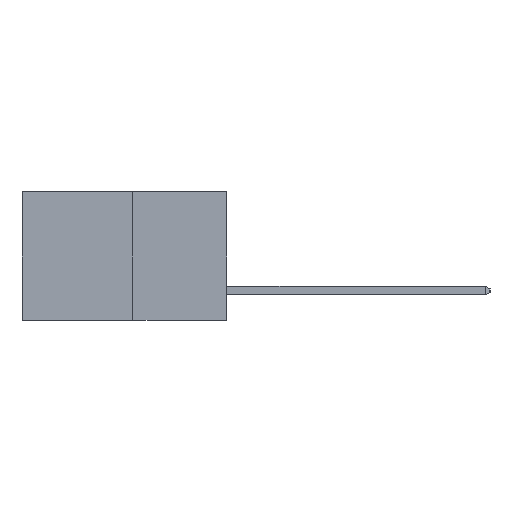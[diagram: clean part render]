
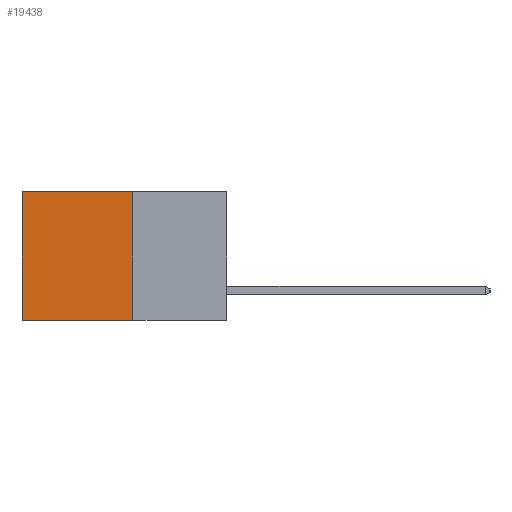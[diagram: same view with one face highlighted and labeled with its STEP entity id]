
A CAD part, left-side view. The second image highlights one B-rep face of the part: STEP entity #19438.
In plain terms, the highlighted planar face has unit normal (-1, 0, 0).
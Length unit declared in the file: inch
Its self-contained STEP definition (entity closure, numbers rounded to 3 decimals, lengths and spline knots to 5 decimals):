
#30 = DIRECTION ( 'NONE',  ( 0., 0., -1. ) ) ;
#348 = DIRECTION ( 'NONE',  ( 0., 1., 0. ) ) ;
#1043 = EDGE_LOOP ( 'NONE', ( #12575, #23502, #5970, #2455 ) ) ;
#2455 = ORIENTED_EDGE ( 'NONE', *, *, #4998, .T. ) ;
#3091 = LINE ( 'NONE', #18232, #7627 ) ;
#3432 = AXIS2_PLACEMENT_3D ( 'NONE', #16353, #6871, #20139 ) ;
#4824 = DIRECTION ( 'NONE',  ( 0., 0., -1. ) ) ;
#4951 = LINE ( 'NONE', #11866, #10711 ) ;
#4998 = EDGE_CURVE ( 'NONE', #17499, #17588, #3091, .T. ) ;
#5282 = EDGE_CURVE ( 'NONE', #17588, #18586, #11205, .T. ) ;
#5970 = ORIENTED_EDGE ( 'NONE', *, *, #10789, .F. ) ;
#6871 = DIRECTION ( 'NONE',  ( 1., 0., 0. ) ) ;
#7493 = VERTEX_POINT ( 'NONE', #19551 ) ;
#7627 = VECTOR ( 'NONE', #8822, 39.37008 ) ;
#8822 = DIRECTION ( 'NONE',  ( 0., 1., 0. ) ) ;
#9646 = CARTESIAN_POINT ( 'NONE',  ( 0.277, 0.59, -0.37 ) ) ;
#10637 = VECTOR ( 'NONE', #30, 39.37008 ) ;
#10711 = VECTOR ( 'NONE', #348, 39.37008 ) ;
#10789 = EDGE_CURVE ( 'NONE', #17499, #7493, #24512, .T. ) ;
#11205 = LINE ( 'NONE', #9646, #10637 ) ;
#11866 = CARTESIAN_POINT ( 'NONE',  ( 0.277, 0.27, -0.37 ) ) ;
#12575 = ORIENTED_EDGE ( 'NONE', *, *, #5282, .T. ) ;
#13930 = VECTOR ( 'NONE', #4824, 39.37008 ) ;
#16353 = CARTESIAN_POINT ( 'NONE',  ( 0.277, 0.27, -0.37 ) ) ;
#17499 = VERTEX_POINT ( 'NONE', #23194 ) ;
#17588 = VERTEX_POINT ( 'NONE', #19754 ) ;
#18155 = CARTESIAN_POINT ( 'NONE',  ( 0.277, 0.27, -0.37 ) ) ;
#18232 = CARTESIAN_POINT ( 'NONE',  ( 0.277, 0.27, 0. ) ) ;
#18586 = VERTEX_POINT ( 'NONE', #22488 ) ;
#19438 = ADVANCED_FACE ( 'NONE', ( #22204 ), #21954, .F. ) ;
#19551 = CARTESIAN_POINT ( 'NONE',  ( 0.277, 0.27, -0.37 ) ) ;
#19754 = CARTESIAN_POINT ( 'NONE',  ( 0.277, 0.59, 0. ) ) ;
#20139 = DIRECTION ( 'NONE',  ( 0., 0., -1. ) ) ;
#20381 = EDGE_CURVE ( 'NONE', #7493, #18586, #4951, .T. ) ;
#21954 = PLANE ( 'NONE',  #3432 ) ;
#22204 = FACE_OUTER_BOUND ( 'NONE', #1043, .T. ) ;
#22488 = CARTESIAN_POINT ( 'NONE',  ( 0.277, 0.59, -0.37 ) ) ;
#23194 = CARTESIAN_POINT ( 'NONE',  ( 0.277, 0.27, 0. ) ) ;
#23502 = ORIENTED_EDGE ( 'NONE', *, *, #20381, .F. ) ;
#24512 = LINE ( 'NONE', #18155, #13930 ) ;
